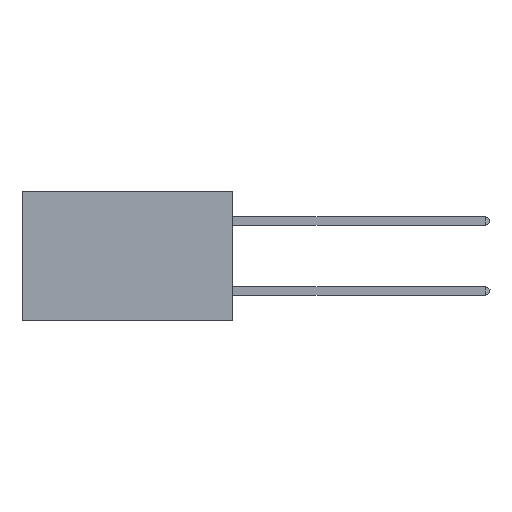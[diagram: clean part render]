
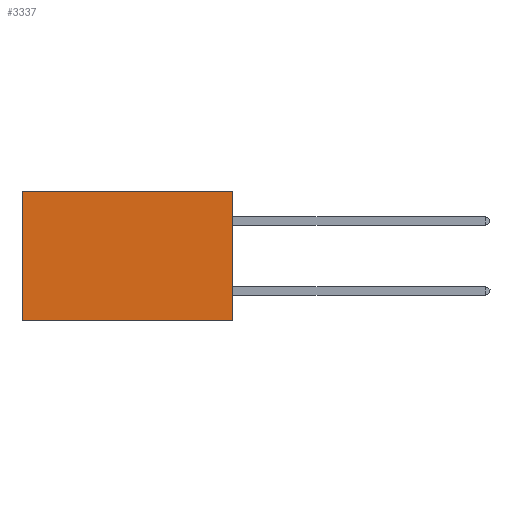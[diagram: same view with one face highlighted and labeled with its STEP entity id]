
A CAD part, left-side view. The second image highlights one B-rep face of the part: STEP entity #3337.
In plain terms, the highlighted planar face has unit normal (-1, 0, 0).
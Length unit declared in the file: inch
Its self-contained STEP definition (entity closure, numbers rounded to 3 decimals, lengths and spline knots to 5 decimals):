
#669 = DIRECTION ( 'NONE',  ( 0., 0., -1. ) ) ;
#721 = VECTOR ( 'NONE', #3646, 39.37008 ) ;
#1309 = VERTEX_POINT ( 'NONE', #10821 ) ;
#1383 = ORIENTED_EDGE ( 'NONE', *, *, #11814, .T. ) ;
#1716 = CARTESIAN_POINT ( 'NONE',  ( 0.2875, 0., 0. ) ) ;
#1873 = FACE_OUTER_BOUND ( 'NONE', #3577, .T. ) ;
#2046 = VECTOR ( 'NONE', #13135, 39.37008 ) ;
#2461 = LINE ( 'NONE', #3355, #721 ) ;
#2568 = DIRECTION ( 'NONE',  ( 1., 0., 0. ) ) ;
#2606 = DIRECTION ( 'NONE',  ( 0., 1., 0. ) ) ;
#2925 = CARTESIAN_POINT ( 'NONE',  ( 0.2875, 0.6, 0. ) ) ;
#3337 = ADVANCED_FACE ( 'NONE', ( #1873 ), #8271, .F. ) ;
#3355 = CARTESIAN_POINT ( 'NONE',  ( 0.2875, 0., 0. ) ) ;
#3577 = EDGE_LOOP ( 'NONE', ( #1383, #12211, #11715, #12451 ) ) ;
#3646 = DIRECTION ( 'NONE',  ( 0., 0., -1. ) ) ;
#4022 = LINE ( 'NONE', #1716, #6062 ) ;
#4396 = LINE ( 'NONE', #2925, #8020 ) ;
#5474 = CARTESIAN_POINT ( 'NONE',  ( 0.2875, 0.6, 0. ) ) ;
#5506 = EDGE_CURVE ( 'NONE', #1309, #6027, #4022, .T. ) ;
#6027 = VERTEX_POINT ( 'NONE', #5474 ) ;
#6047 = CARTESIAN_POINT ( 'NONE',  ( 0.2875, 0., -0.37 ) ) ;
#6062 = VECTOR ( 'NONE', #2606, 39.37008 ) ;
#6458 = VERTEX_POINT ( 'NONE', #8779 ) ;
#6900 = AXIS2_PLACEMENT_3D ( 'NONE', #10494, #2568, #669 ) ;
#7016 = CARTESIAN_POINT ( 'NONE',  ( 0.2875, 0.6, -0.37 ) ) ;
#7248 = EDGE_CURVE ( 'NONE', #1309, #6458, #2461, .T. ) ;
#8020 = VECTOR ( 'NONE', #10015, 39.37008 ) ;
#8049 = LINE ( 'NONE', #6047, #2046 ) ;
#8271 = PLANE ( 'NONE',  #6900 ) ;
#8779 = CARTESIAN_POINT ( 'NONE',  ( 0.2875, 0., -0.37 ) ) ;
#10015 = DIRECTION ( 'NONE',  ( 0., 0., -1. ) ) ;
#10494 = CARTESIAN_POINT ( 'NONE',  ( 0.2875, 0., 0. ) ) ;
#10821 = CARTESIAN_POINT ( 'NONE',  ( 0.2875, 0., 0. ) ) ;
#11020 = VERTEX_POINT ( 'NONE', #7016 ) ;
#11213 = EDGE_CURVE ( 'NONE', #6458, #11020, #8049, .T. ) ;
#11715 = ORIENTED_EDGE ( 'NONE', *, *, #7248, .F. ) ;
#11814 = EDGE_CURVE ( 'NONE', #6027, #11020, #4396, .T. ) ;
#12211 = ORIENTED_EDGE ( 'NONE', *, *, #11213, .F. ) ;
#12451 = ORIENTED_EDGE ( 'NONE', *, *, #5506, .T. ) ;
#13135 = DIRECTION ( 'NONE',  ( 0., 1., 0. ) ) ;
